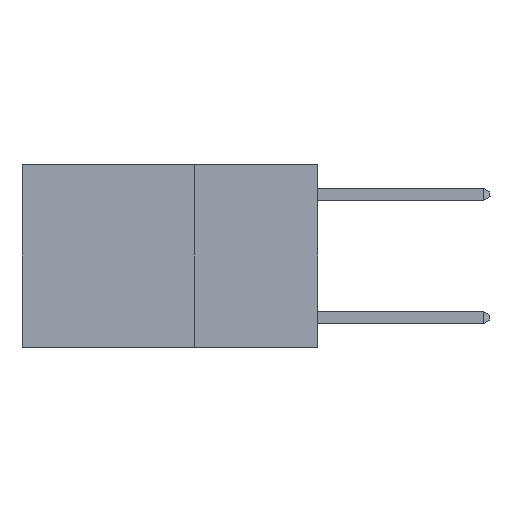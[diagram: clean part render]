
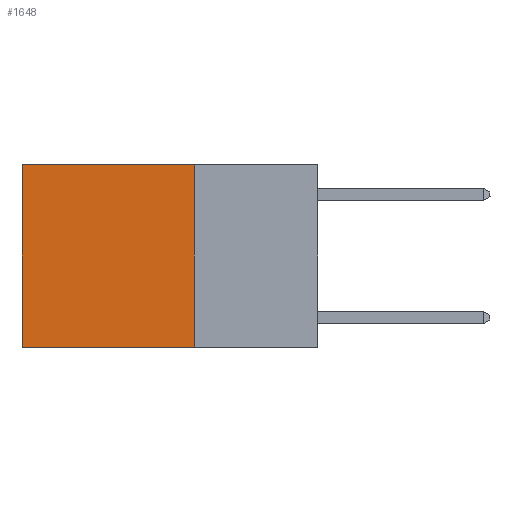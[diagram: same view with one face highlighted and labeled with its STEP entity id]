
A CAD part, left-side view. The second image highlights one B-rep face of the part: STEP entity #1648.
In plain terms, the highlighted planar face has unit normal (-1, 0, 0).
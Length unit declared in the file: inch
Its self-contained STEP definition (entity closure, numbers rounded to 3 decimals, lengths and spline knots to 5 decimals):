
#5 = PLANE ( 'NONE',  #18282 ) ;
#1015 = VECTOR ( 'NONE', #5039, 39.37008 ) ;
#1144 = VERTEX_POINT ( 'NONE', #28658 ) ;
#1648 = ADVANCED_FACE ( 'NONE', ( #19364 ), #5, .F. ) ;
#1733 = LINE ( 'NONE', #9713, #1015 ) ;
#2201 = DIRECTION ( 'NONE',  ( 0., 0., -1. ) ) ;
#2381 = ORIENTED_EDGE ( 'NONE', *, *, #15270, .F. ) ;
#2437 = CARTESIAN_POINT ( 'NONE',  ( 0.2625, 0.25, 0. ) ) ;
#3828 = LINE ( 'NONE', #7045, #14966 ) ;
#5039 = DIRECTION ( 'NONE',  ( 0., 1., 0. ) ) ;
#5180 = DIRECTION ( 'NONE',  ( 0., 1., 0. ) ) ;
#5330 = CARTESIAN_POINT ( 'NONE',  ( 0.2625, 0.25, 0. ) ) ;
#6854 = EDGE_CURVE ( 'NONE', #14417, #1144, #1733, .T. ) ;
#7045 = CARTESIAN_POINT ( 'NONE',  ( 0.2625, 0.25, -0.37 ) ) ;
#7093 = DIRECTION ( 'NONE',  ( 0., 0., -1. ) ) ;
#7189 = CARTESIAN_POINT ( 'NONE',  ( 0.2625, 0.6, 0. ) ) ;
#9360 = EDGE_CURVE ( 'NONE', #1144, #19614, #15353, .T. ) ;
#9713 = CARTESIAN_POINT ( 'NONE',  ( 0.2625, 0.25, 0. ) ) ;
#10069 = CARTESIAN_POINT ( 'NONE',  ( 0.2625, 0.25, -0.37 ) ) ;
#10076 = EDGE_CURVE ( 'NONE', #11593, #19614, #3828, .T. ) ;
#11593 = VERTEX_POINT ( 'NONE', #10069 ) ;
#12190 = CARTESIAN_POINT ( 'NONE',  ( 0.2625, 0.6, -0.37 ) ) ;
#13621 = CARTESIAN_POINT ( 'NONE',  ( 0.2625, 0.25, 0. ) ) ;
#14417 = VERTEX_POINT ( 'NONE', #5330 ) ;
#14966 = VECTOR ( 'NONE', #5180, 39.37008 ) ;
#15270 = EDGE_CURVE ( 'NONE', #14417, #11593, #21704, .T. ) ;
#15353 = LINE ( 'NONE', #7189, #21406 ) ;
#16487 = EDGE_LOOP ( 'NONE', ( #17976, #21306, #2381, #17645 ) ) ;
#16992 = VECTOR ( 'NONE', #2201, 39.37008 ) ;
#17645 = ORIENTED_EDGE ( 'NONE', *, *, #6854, .T. ) ;
#17976 = ORIENTED_EDGE ( 'NONE', *, *, #9360, .T. ) ;
#18282 = AXIS2_PLACEMENT_3D ( 'NONE', #2437, #23357, #27544 ) ;
#19364 = FACE_OUTER_BOUND ( 'NONE', #16487, .T. ) ;
#19614 = VERTEX_POINT ( 'NONE', #12190 ) ;
#21306 = ORIENTED_EDGE ( 'NONE', *, *, #10076, .F. ) ;
#21406 = VECTOR ( 'NONE', #7093, 39.37008 ) ;
#21704 = LINE ( 'NONE', #13621, #16992 ) ;
#23357 = DIRECTION ( 'NONE',  ( 1., 0., 0. ) ) ;
#27544 = DIRECTION ( 'NONE',  ( 0., 0., -1. ) ) ;
#28658 = CARTESIAN_POINT ( 'NONE',  ( 0.2625, 0.6, 0. ) ) ;
